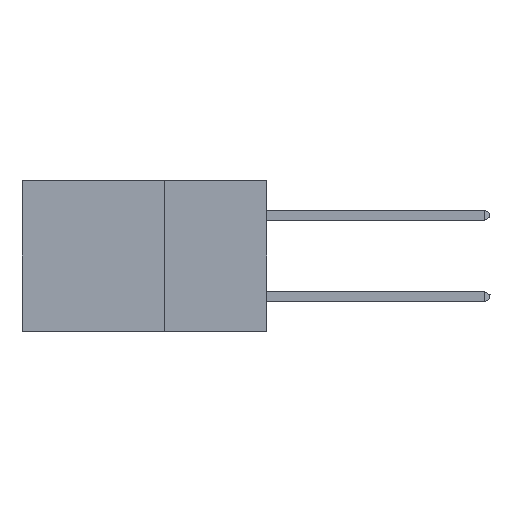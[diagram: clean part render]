
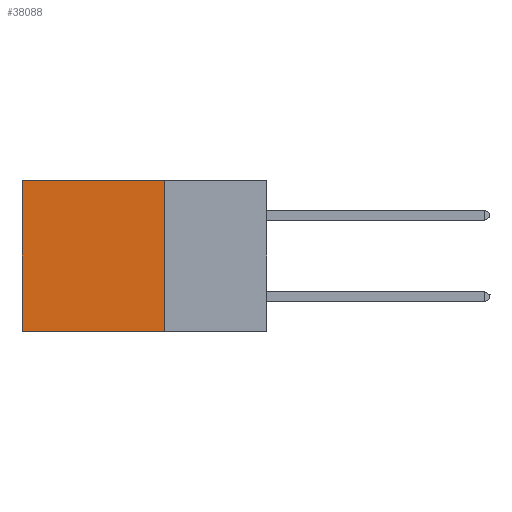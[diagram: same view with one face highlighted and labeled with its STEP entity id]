
A CAD part, left-side view. The second image highlights one B-rep face of the part: STEP entity #38088.
In plain terms, the highlighted planar face has unit normal (-1, 0, 0).
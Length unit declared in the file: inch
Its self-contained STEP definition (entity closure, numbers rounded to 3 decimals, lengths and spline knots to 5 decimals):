
#2281 = FACE_OUTER_BOUND ( 'NONE', #4851, .T. ) ;
#3911 = CARTESIAN_POINT ( 'NONE',  ( 0.2875, 0.25, -0.37 ) ) ;
#4745 = CARTESIAN_POINT ( 'NONE',  ( 0.2875, 0.25, 0. ) ) ;
#4851 = EDGE_LOOP ( 'NONE', ( #9553, #10397, #29126, #11845 ) ) ;
#6632 = DIRECTION ( 'NONE',  ( 0., 0., -1. ) ) ;
#8409 = EDGE_CURVE ( 'NONE', #34523, #19011, #34425, .T. ) ;
#8757 = VECTOR ( 'NONE', #12006, 39.37008 ) ;
#9553 = ORIENTED_EDGE ( 'NONE', *, *, #17565, .T. ) ;
#10397 = ORIENTED_EDGE ( 'NONE', *, *, #15632, .F. ) ;
#11845 = ORIENTED_EDGE ( 'NONE', *, *, #8409, .T. ) ;
#12006 = DIRECTION ( 'NONE',  ( 0., 0., -1. ) ) ;
#15326 = VERTEX_POINT ( 'NONE', #20851 ) ;
#15632 = EDGE_CURVE ( 'NONE', #33116, #15326, #35572, .T. ) ;
#17565 = EDGE_CURVE ( 'NONE', #19011, #15326, #29505, .T. ) ;
#19011 = VERTEX_POINT ( 'NONE', #34214 ) ;
#20769 = DIRECTION ( 'NONE',  ( 0., 0., -1. ) ) ;
#20851 = CARTESIAN_POINT ( 'NONE',  ( 0.2875, 0.6, -0.37 ) ) ;
#21478 = VECTOR ( 'NONE', #34229, 39.37008 ) ;
#21633 = VECTOR ( 'NONE', #6632, 39.37008 ) ;
#22265 = LINE ( 'NONE', #25537, #21633 ) ;
#25537 = CARTESIAN_POINT ( 'NONE',  ( 0.2875, 0.25, 0. ) ) ;
#27339 = DIRECTION ( 'NONE',  ( 1., 0., 0. ) ) ;
#29126 = ORIENTED_EDGE ( 'NONE', *, *, #29511, .F. ) ;
#29170 = CARTESIAN_POINT ( 'NONE',  ( 0.2875, 0.25, -0.37 ) ) ;
#29505 = LINE ( 'NONE', #30713, #8757 ) ;
#29511 = EDGE_CURVE ( 'NONE', #34523, #33116, #22265, .T. ) ;
#30541 = AXIS2_PLACEMENT_3D ( 'NONE', #4745, #27339, #20769 ) ;
#30713 = CARTESIAN_POINT ( 'NONE',  ( 0.2875, 0.6, 0. ) ) ;
#32910 = PLANE ( 'NONE',  #30541 ) ;
#32973 = VECTOR ( 'NONE', #35970, 39.37008 ) ;
#33116 = VERTEX_POINT ( 'NONE', #29170 ) ;
#33954 = CARTESIAN_POINT ( 'NONE',  ( 0.2875, 0.25, 0. ) ) ;
#34057 = CARTESIAN_POINT ( 'NONE',  ( 0.2875, 0.25, 0. ) ) ;
#34214 = CARTESIAN_POINT ( 'NONE',  ( 0.2875, 0.6, 0. ) ) ;
#34229 = DIRECTION ( 'NONE',  ( 0., 1., 0. ) ) ;
#34425 = LINE ( 'NONE', #34057, #21478 ) ;
#34523 = VERTEX_POINT ( 'NONE', #33954 ) ;
#35572 = LINE ( 'NONE', #3911, #32973 ) ;
#35970 = DIRECTION ( 'NONE',  ( 0., 1., 0. ) ) ;
#38088 = ADVANCED_FACE ( 'NONE', ( #2281 ), #32910, .F. ) ;
